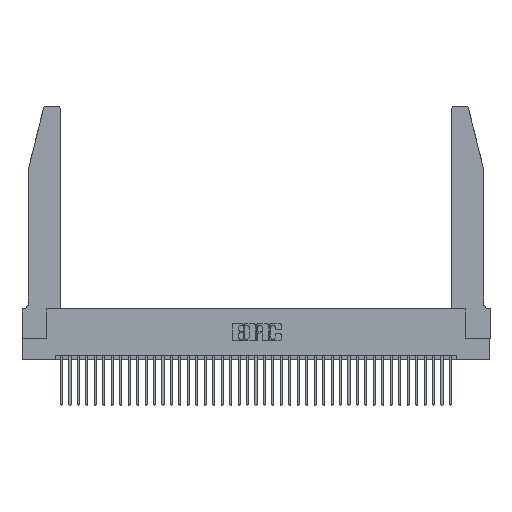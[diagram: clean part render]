
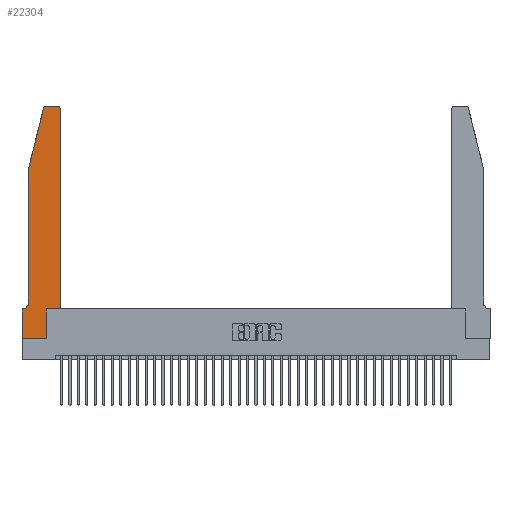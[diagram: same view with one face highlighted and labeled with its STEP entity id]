
A CAD part, top view. The second image highlights one B-rep face of the part: STEP entity #22304.
In plain terms, the highlighted planar face has unit normal (0, 0, 1).
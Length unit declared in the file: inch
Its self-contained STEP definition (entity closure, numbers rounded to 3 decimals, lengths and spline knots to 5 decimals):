
#365 = CARTESIAN_POINT ( 'NONE',  ( 0.284, 2.75, 0.37 ) ) ;
#453 = LINE ( 'NONE', #17384, #17523 ) ;
#757 = VERTEX_POINT ( 'NONE', #19839 ) ;
#1073 = CARTESIAN_POINT ( 'NONE',  ( 0.0055, 0.35, 0.37 ) ) ;
#1221 = VECTOR ( 'NONE', #8557, 39.37008 ) ;
#1594 = LINE ( 'NONE', #36041, #9206 ) ;
#1864 = DIRECTION ( 'NONE',  ( 1., 0., 0. ) ) ;
#2289 = CIRCLE ( 'NONE', #25252, 0.03 ) ;
#2364 = CARTESIAN_POINT ( 'NONE',  ( 0.4505, 0.35, 0.37 ) ) ;
#2470 = DIRECTION ( 'NONE',  ( -1., 0., 0. ) ) ;
#2758 = CARTESIAN_POINT ( 'NONE',  ( 0., 0.35, 0.37 ) ) ;
#2925 = EDGE_CURVE ( 'NONE', #12358, #3136, #31344, .T. ) ;
#2988 = EDGE_CURVE ( 'NONE', #27287, #36349, #29371, .T. ) ;
#3136 = VERTEX_POINT ( 'NONE', #365 ) ;
#3419 = EDGE_CURVE ( 'NONE', #36349, #14117, #30322, .T. ) ;
#3442 = CARTESIAN_POINT ( 'NONE',  ( 0.0755, 2., 0.37 ) ) ;
#3661 = EDGE_CURVE ( 'NONE', #14171, #30995, #30810, .T. ) ;
#3946 = EDGE_CURVE ( 'NONE', #29947, #27287, #38182, .T. ) ;
#4295 = DIRECTION ( 'NONE',  ( 0., 1., 0. ) ) ;
#4468 = EDGE_CURVE ( 'NONE', #14117, #5062, #36764, .T. ) ;
#4879 = DIRECTION ( 'NONE',  ( -1., 0., 0. ) ) ;
#5062 = VERTEX_POINT ( 'NONE', #16365 ) ;
#5275 = CARTESIAN_POINT ( 'NONE',  ( 0.4505, 0.35, 0.37 ) ) ;
#6127 = CARTESIAN_POINT ( 'NONE',  ( 0.2865, 0., 0.37 ) ) ;
#6593 = DIRECTION ( 'NONE',  ( 0., 0., 1. ) ) ;
#7022 = DIRECTION ( 'NONE',  ( -0.239, -0.971, 0. ) ) ;
#7221 = AXIS2_PLACEMENT_3D ( 'NONE', #8677, #30820, #11924 ) ;
#7501 = CIRCLE ( 'NONE', #7221, 0.03 ) ;
#7683 = ORIENTED_EDGE ( 'NONE', *, *, #3419, .T. ) ;
#7953 = CIRCLE ( 'NONE', #12141, 0.07 ) ;
#8099 = EDGE_CURVE ( 'NONE', #5062, #29536, #26657, .T. ) ;
#8557 = DIRECTION ( 'NONE',  ( 1., 0., 0. ) ) ;
#8677 = CARTESIAN_POINT ( 'NONE',  ( 0.284, 2.72, 0.37 ) ) ;
#9206 = VECTOR ( 'NONE', #4295, 39.37008 ) ;
#9404 = DIRECTION ( 'NONE',  ( 0., -1., 0. ) ) ;
#10390 = CARTESIAN_POINT ( 'NONE',  ( 0.2865, 0.35, 0.37 ) ) ;
#10425 = DIRECTION ( 'NONE',  ( 1., 0., 0. ) ) ;
#11661 = VECTOR ( 'NONE', #32610, 39.37008 ) ;
#11924 = DIRECTION ( 'NONE',  ( 1., 0., 0. ) ) ;
#12097 = CARTESIAN_POINT ( 'NONE',  ( 0.2605, 2.75, 0.37 ) ) ;
#12141 = AXIS2_PLACEMENT_3D ( 'NONE', #12439, #34441, #15649 ) ;
#12358 = VERTEX_POINT ( 'NONE', #13163 ) ;
#12439 = CARTESIAN_POINT ( 'NONE',  ( 0.0055, 0.42, 0.37 ) ) ;
#12782 = EDGE_CURVE ( 'NONE', #3136, #14171, #7501, .T. ) ;
#13116 = ORIENTED_EDGE ( 'NONE', *, *, #2988, .T. ) ;
#13163 = CARTESIAN_POINT ( 'NONE',  ( 0.4205, 2.75, 0.37 ) ) ;
#13480 = EDGE_CURVE ( 'NONE', #17578, #29947, #7953, .T. ) ;
#14117 = VERTEX_POINT ( 'NONE', #6127 ) ;
#14171 = VERTEX_POINT ( 'NONE', #19138 ) ;
#14465 = AXIS2_PLACEMENT_3D ( 'NONE', #26177, #29351, #10425 ) ;
#15476 = ORIENTED_EDGE ( 'NONE', *, *, #12782, .T. ) ;
#15649 = DIRECTION ( 'NONE',  ( -1., 0., 0. ) ) ;
#16117 = CARTESIAN_POINT ( 'NONE',  ( 0.0755, 0.42, 0.37 ) ) ;
#16365 = CARTESIAN_POINT ( 'NONE',  ( 0.2865, 0.35, 0.37 ) ) ;
#16686 = ORIENTED_EDGE ( 'NONE', *, *, #36153, .T. ) ;
#17384 = CARTESIAN_POINT ( 'NONE',  ( 0.0755, 2., 0.37 ) ) ;
#17503 = ORIENTED_EDGE ( 'NONE', *, *, #37926, .T. ) ;
#17523 = VECTOR ( 'NONE', #39314, 39.37008 ) ;
#17578 = VERTEX_POINT ( 'NONE', #16117 ) ;
#18091 = ORIENTED_EDGE ( 'NONE', *, *, #30416, .T. ) ;
#18866 = ORIENTED_EDGE ( 'NONE', *, *, #3661, .T. ) ;
#19138 = CARTESIAN_POINT ( 'NONE',  ( 0.25487, 2.72718, 0.37 ) ) ;
#19839 = CARTESIAN_POINT ( 'NONE',  ( 0.4505, 2.72, 0.37 ) ) ;
#20451 = ORIENTED_EDGE ( 'NONE', *, *, #3946, .T. ) ;
#20663 = FACE_OUTER_BOUND ( 'NONE', #27929, .T. ) ;
#21022 = CARTESIAN_POINT ( 'NONE',  ( 0., 0., 0.37 ) ) ;
#22304 = ADVANCED_FACE ( 'NONE', ( #20663 ), #23023, .T. ) ;
#22435 = VECTOR ( 'NONE', #7022, 39.37008 ) ;
#22982 = VECTOR ( 'NONE', #2470, 39.37008 ) ;
#23023 = PLANE ( 'NONE',  #14465 ) ;
#23996 = CARTESIAN_POINT ( 'NONE',  ( 0.0755, 0.35, 0.37 ) ) ;
#25252 = AXIS2_PLACEMENT_3D ( 'NONE', #25655, #6593, #28802 ) ;
#25655 = CARTESIAN_POINT ( 'NONE',  ( 0.4205, 2.72, 0.37 ) ) ;
#26069 = CARTESIAN_POINT ( 'NONE',  ( 0.0755, 2., 0.37 ) ) ;
#26177 = CARTESIAN_POINT ( 'NONE',  ( 0., 0.35, 0.37 ) ) ;
#26657 = LINE ( 'NONE', #5275, #1221 ) ;
#27287 = VERTEX_POINT ( 'NONE', #2758 ) ;
#27929 = EDGE_LOOP ( 'NONE', ( #28015, #15476, #18866, #17503, #32198, #20451, #13116, #7683, #39880, #39100, #16686, #18091 ) ) ;
#28015 = ORIENTED_EDGE ( 'NONE', *, *, #2925, .T. ) ;
#28802 = DIRECTION ( 'NONE',  ( 1., 0., 0. ) ) ;
#29351 = DIRECTION ( 'NONE',  ( 0., 0., 1. ) ) ;
#29371 = LINE ( 'NONE', #34644, #37693 ) ;
#29463 = VECTOR ( 'NONE', #4879, 39.37008 ) ;
#29536 = VERTEX_POINT ( 'NONE', #2364 ) ;
#29947 = VERTEX_POINT ( 'NONE', #1073 ) ;
#30322 = LINE ( 'NONE', #21022, #38619 ) ;
#30416 = EDGE_CURVE ( 'NONE', #757, #12358, #2289, .T. ) ;
#30810 = LINE ( 'NONE', #26069, #22435 ) ;
#30820 = DIRECTION ( 'NONE',  ( 0., 0., 1. ) ) ;
#30995 = VERTEX_POINT ( 'NONE', #3442 ) ;
#31344 = LINE ( 'NONE', #12097, #22982 ) ;
#32198 = ORIENTED_EDGE ( 'NONE', *, *, #13480, .T. ) ;
#32610 = DIRECTION ( 'NONE',  ( 0., 1., 0. ) ) ;
#34441 = DIRECTION ( 'NONE',  ( 0., 0., -1. ) ) ;
#34644 = CARTESIAN_POINT ( 'NONE',  ( 0., 0., 0.37 ) ) ;
#36041 = CARTESIAN_POINT ( 'NONE',  ( 0.4505, 0.35, 0.37 ) ) ;
#36153 = EDGE_CURVE ( 'NONE', #29536, #757, #1594, .T. ) ;
#36349 = VERTEX_POINT ( 'NONE', #39986 ) ;
#36764 = LINE ( 'NONE', #10390, #11661 ) ;
#37693 = VECTOR ( 'NONE', #9404, 39.37008 ) ;
#37926 = EDGE_CURVE ( 'NONE', #30995, #17578, #453, .T. ) ;
#38182 = LINE ( 'NONE', #23996, #29463 ) ;
#38619 = VECTOR ( 'NONE', #1864, 39.37008 ) ;
#39100 = ORIENTED_EDGE ( 'NONE', *, *, #8099, .T. ) ;
#39314 = DIRECTION ( 'NONE',  ( 0., -1., 0. ) ) ;
#39880 = ORIENTED_EDGE ( 'NONE', *, *, #4468, .T. ) ;
#39986 = CARTESIAN_POINT ( 'NONE',  ( 0., 0., 0.37 ) ) ;
